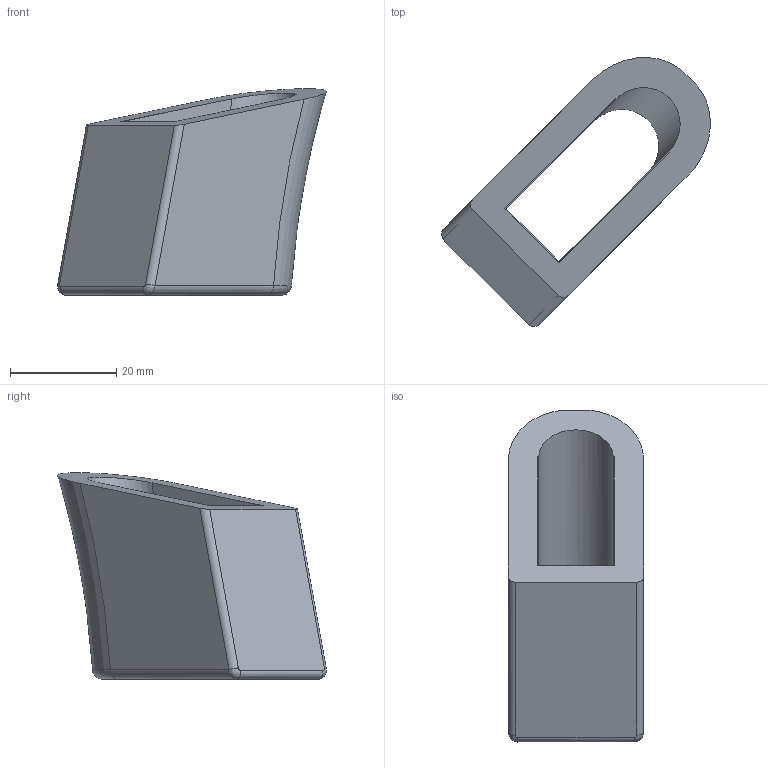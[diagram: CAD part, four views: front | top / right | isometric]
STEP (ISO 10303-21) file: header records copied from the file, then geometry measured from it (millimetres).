
FILE_DESCRIPTION(/* description */ (''),/* implementation_level */ '2;1');
FILE_NAME(/* name */ 'mag grip.step',/* time_stamp */ '2021-09-02T19:32:50-05:00',/* author */ (''),/* organization */ (''),/* preprocessor_version */ 'ST-DEVELOPER v18.1',/* originating_system */ 'Autodesk Translation Framework v10.10.0.1391',/* authorisation */ '');
FILE_SCHEMA (('AUTOMOTIVE_DESIGN { 1 0 10303 214 3 1 1 }'));
Length unit declared in the file: millimetre
Products named in the file (1): mag grip
Bounding box: 50.51 x 50.54 x 38.77 mm (x, y, z)
Volume: 19599.6 mm3; surface area: 8801.2 mm2
Topology: 1 solids, 1 shells, 46 faces, 124 edges, 77 vertices
Faces by surface type: plane 22, cylinder 11, cone 5, torus 4, sphere 2, bspline 2
Entity records: 2316 total; most frequent: CARTESIAN_POINT 1203, ORIENTED_EDGE 244, DIRECTION 193, EDGE_CURVE 122, VERTEX_POINT 77, AXIS2_PLACEMENT_3D 65, LINE 63, VECTOR 63
